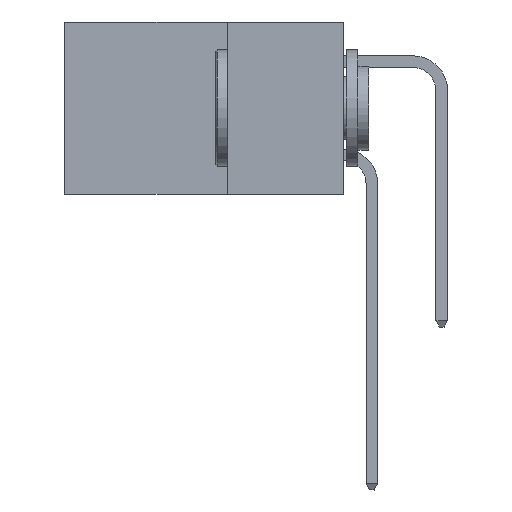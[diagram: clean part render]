
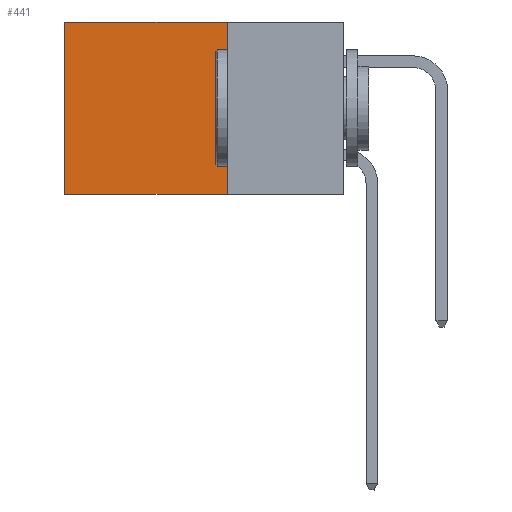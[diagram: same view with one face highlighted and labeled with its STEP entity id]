
A CAD part, left-side view. The second image highlights one B-rep face of the part: STEP entity #441.
In plain terms, the highlighted planar face has unit normal (-1, 0, 0).
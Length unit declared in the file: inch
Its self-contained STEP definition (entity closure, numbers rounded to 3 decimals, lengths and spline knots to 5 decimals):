
#299 = DIRECTION ( 'NONE',  ( 0., 1., 0. ) ) ;
#441 = ADVANCED_FACE ( 'NONE', ( #21479 ), #31243, .F. ) ;
#667 = ORIENTED_EDGE ( 'NONE', *, *, #26281, .T. ) ;
#2186 = CARTESIAN_POINT ( 'NONE',  ( 0.298, 0.6, 0. ) ) ;
#2285 = VERTEX_POINT ( 'NONE', #2186 ) ;
#4203 = EDGE_CURVE ( 'NONE', #21916, #14752, #10154, .T. ) ;
#4405 = CARTESIAN_POINT ( 'NONE',  ( 0.298, 0.25, 0. ) ) ;
#4756 = VECTOR ( 'NONE', #19362, 39.37008 ) ;
#5514 = LINE ( 'NONE', #31236, #31781 ) ;
#7517 = AXIS2_PLACEMENT_3D ( 'NONE', #23714, #13786, #8714 ) ;
#8714 = DIRECTION ( 'NONE',  ( 0., 0., -1. ) ) ;
#9528 = CARTESIAN_POINT ( 'NONE',  ( 0.298, 0.6, -0.37 ) ) ;
#10154 = LINE ( 'NONE', #22890, #10570 ) ;
#10570 = VECTOR ( 'NONE', #299, 39.37008 ) ;
#13786 = DIRECTION ( 'NONE',  ( 1., 0., 0. ) ) ;
#14752 = VERTEX_POINT ( 'NONE', #9528 ) ;
#15003 = EDGE_CURVE ( 'NONE', #23076, #21916, #20915, .T. ) ;
#15142 = ORIENTED_EDGE ( 'NONE', *, *, #15003, .F. ) ;
#16189 = DIRECTION ( 'NONE',  ( 0., 0., -1. ) ) ;
#18871 = LINE ( 'NONE', #22028, #4756 ) ;
#19318 = VECTOR ( 'NONE', #29595, 39.37008 ) ;
#19362 = DIRECTION ( 'NONE',  ( 0., 1., 0. ) ) ;
#19534 = CARTESIAN_POINT ( 'NONE',  ( 0.298, 0.25, 0. ) ) ;
#20915 = LINE ( 'NONE', #19534, #19318 ) ;
#21479 = FACE_OUTER_BOUND ( 'NONE', #22415, .T. ) ;
#21916 = VERTEX_POINT ( 'NONE', #26242 ) ;
#22028 = CARTESIAN_POINT ( 'NONE',  ( 0.298, 0.25, 0. ) ) ;
#22415 = EDGE_LOOP ( 'NONE', ( #24818, #29942, #15142, #667 ) ) ;
#22890 = CARTESIAN_POINT ( 'NONE',  ( 0.298, 0.25, -0.37 ) ) ;
#23076 = VERTEX_POINT ( 'NONE', #4405 ) ;
#23714 = CARTESIAN_POINT ( 'NONE',  ( 0.298, 0.25, 0. ) ) ;
#23883 = EDGE_CURVE ( 'NONE', #2285, #14752, #5514, .T. ) ;
#24818 = ORIENTED_EDGE ( 'NONE', *, *, #23883, .T. ) ;
#26242 = CARTESIAN_POINT ( 'NONE',  ( 0.298, 0.25, -0.37 ) ) ;
#26281 = EDGE_CURVE ( 'NONE', #23076, #2285, #18871, .T. ) ;
#29595 = DIRECTION ( 'NONE',  ( 0., 0., -1. ) ) ;
#29942 = ORIENTED_EDGE ( 'NONE', *, *, #4203, .F. ) ;
#31236 = CARTESIAN_POINT ( 'NONE',  ( 0.298, 0.6, 0. ) ) ;
#31243 = PLANE ( 'NONE',  #7517 ) ;
#31781 = VECTOR ( 'NONE', #16189, 39.37008 ) ;
